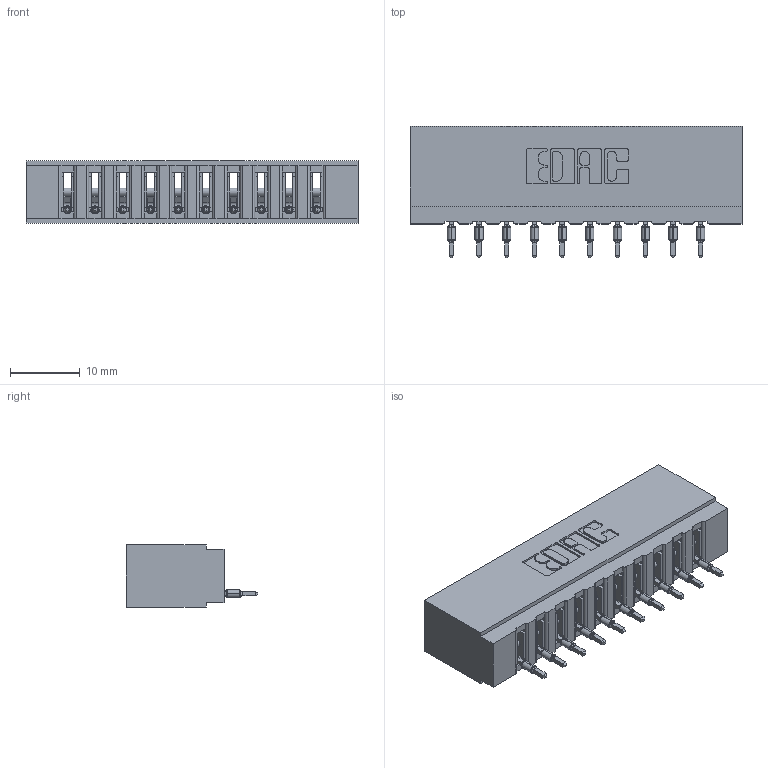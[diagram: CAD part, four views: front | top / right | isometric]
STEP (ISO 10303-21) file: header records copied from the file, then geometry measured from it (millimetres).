
FILE_DESCRIPTION (( 'STEP AP203' ), '1' );
FILE_NAME ('717-010-560-106.STEP', '2020-03-13T18:01:01', ( '' ), ( '' ), 'SwSTEP 2.0', 'SolidWorks 2016', '' );
FILE_SCHEMA (( 'CONFIG_CONTROL_DESIGN' ));
Length unit declared in the file: inch
Products named in the file (3): 745-292-001_560; 717-010-560-106; 717 Part_Insulator Option - 06
Assembly tree (11 placements, depth 2):
  717-010-560-106
    717 Part_Insulator Option - 06
    745-292-001_560  x10
Bounding box: 47.5 x 18.78 x 8.89 mm (x, y, z)
Volume: 4187 mm3; surface area: 5695.4 mm2
Topology: 11 solids, 11 shells, 1314 faces, 3651 edges, 2326 vertices
Faces by surface type: plane 784, cylinder 270, bspline 200, torus 60
Entity records: 21474 total; most frequent: CARTESIAN_POINT 4285, ORIENTED_EDGE 3666, DIRECTION 3215, EDGE_CURVE 1833, VECTOR 1583, LINE 1583, VERTEX_POINT 1174, AXIS2_PLACEMENT_3D 816
